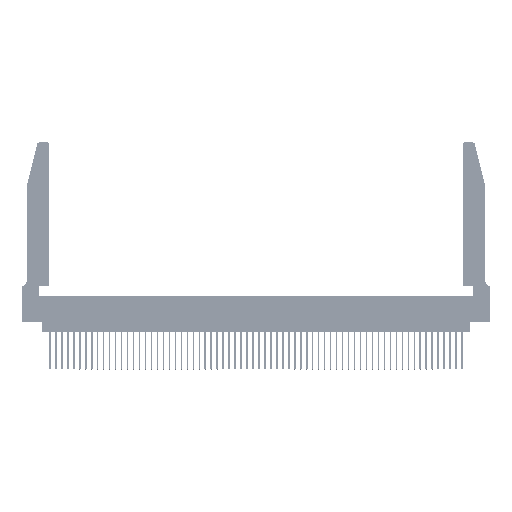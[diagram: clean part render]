
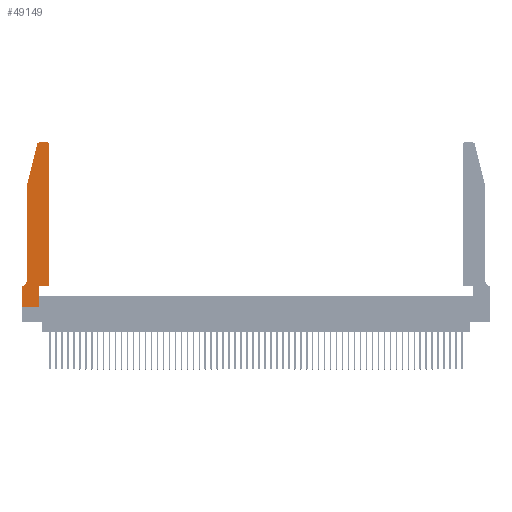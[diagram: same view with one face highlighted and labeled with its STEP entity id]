
A CAD part, top view. The second image highlights one B-rep face of the part: STEP entity #49149.
In plain terms, the highlighted planar face has unit normal (0, 0, 1).
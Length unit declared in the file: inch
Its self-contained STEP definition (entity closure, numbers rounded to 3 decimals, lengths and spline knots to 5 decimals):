
#308 = LINE ( 'NONE', #42443, #46411 ) ;
#454 = EDGE_CURVE ( 'NONE', #34632, #51511, #42920, .T. ) ;
#538 = LINE ( 'NONE', #3701, #51428 ) ;
#749 = EDGE_CURVE ( 'NONE', #15492, #6159, #21286, .T. ) ;
#1790 = CARTESIAN_POINT ( 'NONE',  ( 0.4205, 2.72, 0.37 ) ) ;
#1946 = DIRECTION ( 'NONE',  ( 1., 0., 0. ) ) ;
#1961 = VECTOR ( 'NONE', #26047, 39.37008 ) ;
#2184 = AXIS2_PLACEMENT_3D ( 'NONE', #32062, #45126, #1946 ) ;
#2428 = CARTESIAN_POINT ( 'NONE',  ( 0., 0.35, 0.37 ) ) ;
#2936 = FACE_OUTER_BOUND ( 'NONE', #8441, .T. ) ;
#3701 = CARTESIAN_POINT ( 'NONE',  ( 0., 0., 0.37 ) ) ;
#4046 = ORIENTED_EDGE ( 'NONE', *, *, #21004, .T. ) ;
#4963 = DIRECTION ( 'NONE',  ( -1., 0., 0. ) ) ;
#6159 = VERTEX_POINT ( 'NONE', #52684 ) ;
#6370 = VERTEX_POINT ( 'NONE', #18988 ) ;
#6462 = CIRCLE ( 'NONE', #9259, 0.03 ) ;
#6518 = ORIENTED_EDGE ( 'NONE', *, *, #55956, .T. ) ;
#6593 = CIRCLE ( 'NONE', #7332, 0.07 ) ;
#7332 = AXIS2_PLACEMENT_3D ( 'NONE', #45254, #49633, #28563 ) ;
#8377 = CARTESIAN_POINT ( 'NONE',  ( 0.0755, 2., 0.37 ) ) ;
#8441 = EDGE_LOOP ( 'NONE', ( #33001, #18082, #33596, #13042, #40337, #54365, #6518, #4046, #44190, #26264, #25350, #10329 ) ) ;
#9259 = AXIS2_PLACEMENT_3D ( 'NONE', #1790, #28641, #28462 ) ;
#10329 = ORIENTED_EDGE ( 'NONE', *, *, #38679, .T. ) ;
#11147 = VERTEX_POINT ( 'NONE', #2428 ) ;
#12492 = CARTESIAN_POINT ( 'NONE',  ( 0.0755, 2., 0.37 ) ) ;
#13042 = ORIENTED_EDGE ( 'NONE', *, *, #749, .T. ) ;
#13101 = EDGE_CURVE ( 'NONE', #50564, #11147, #18239, .T. ) ;
#14091 = DIRECTION ( 'NONE',  ( 0., 0., 1. ) ) ;
#14853 = CARTESIAN_POINT ( 'NONE',  ( 0.0755, 2., 0.37 ) ) ;
#15492 = VERTEX_POINT ( 'NONE', #12492 ) ;
#17785 = CARTESIAN_POINT ( 'NONE',  ( 0.4505, 0.35, 0.37 ) ) ;
#17996 = AXIS2_PLACEMENT_3D ( 'NONE', #18849, #14091, #49141 ) ;
#18082 = ORIENTED_EDGE ( 'NONE', *, *, #454, .T. ) ;
#18239 = LINE ( 'NONE', #39400, #41235 ) ;
#18849 = CARTESIAN_POINT ( 'NONE',  ( 0.284, 2.72, 0.37 ) ) ;
#18988 = CARTESIAN_POINT ( 'NONE',  ( 0.2865, 0.35, 0.37 ) ) ;
#20338 = DIRECTION ( 'NONE',  ( 0., 1., 0. ) ) ;
#21004 = EDGE_CURVE ( 'NONE', #37998, #21715, #23641, .T. ) ;
#21286 = LINE ( 'NONE', #8377, #32148 ) ;
#21448 = CARTESIAN_POINT ( 'NONE',  ( 0.4505, 2.72, 0.37 ) ) ;
#21715 = VERTEX_POINT ( 'NONE', #52553 ) ;
#23641 = LINE ( 'NONE', #29854, #1961 ) ;
#23735 = DIRECTION ( 'NONE',  ( -0.239, -0.971, 0. ) ) ;
#24909 = LINE ( 'NONE', #42332, #50003 ) ;
#25350 = ORIENTED_EDGE ( 'NONE', *, *, #33210, .T. ) ;
#25373 = CARTESIAN_POINT ( 'NONE',  ( 0.4205, 2.75, 0.37 ) ) ;
#25662 = VERTEX_POINT ( 'NONE', #25373 ) ;
#26047 = DIRECTION ( 'NONE',  ( 1., 0., 0. ) ) ;
#26264 = ORIENTED_EDGE ( 'NONE', *, *, #28695, .T. ) ;
#26743 = LINE ( 'NONE', #14853, #49842 ) ;
#28462 = DIRECTION ( 'NONE',  ( 1., 0., 0. ) ) ;
#28563 = DIRECTION ( 'NONE',  ( -1., 0., 0. ) ) ;
#28641 = DIRECTION ( 'NONE',  ( 0., 0., 1. ) ) ;
#28695 = EDGE_CURVE ( 'NONE', #6370, #44546, #34144, .T. ) ;
#29854 = CARTESIAN_POINT ( 'NONE',  ( 0., 0., 0.37 ) ) ;
#29981 = DIRECTION ( 'NONE',  ( 0., -1., 0. ) ) ;
#30315 = DIRECTION ( 'NONE',  ( 0., -1., 0. ) ) ;
#31941 = LINE ( 'NONE', #37715, #55636 ) ;
#32062 = CARTESIAN_POINT ( 'NONE',  ( 0., 0.35, 0.37 ) ) ;
#32148 = VECTOR ( 'NONE', #30315, 39.37008 ) ;
#32847 = DIRECTION ( 'NONE',  ( 1., 0., 0. ) ) ;
#33001 = ORIENTED_EDGE ( 'NONE', *, *, #38830, .T. ) ;
#33210 = EDGE_CURVE ( 'NONE', #44546, #39086, #24909, .T. ) ;
#33596 = ORIENTED_EDGE ( 'NONE', *, *, #38611, .T. ) ;
#33680 = CARTESIAN_POINT ( 'NONE',  ( 0.284, 2.75, 0.37 ) ) ;
#33989 = DIRECTION ( 'NONE',  ( 0., 1., 0. ) ) ;
#34144 = LINE ( 'NONE', #54081, #54491 ) ;
#34632 = VERTEX_POINT ( 'NONE', #33680 ) ;
#35718 = CARTESIAN_POINT ( 'NONE',  ( 0., 0., 0.37 ) ) ;
#37715 = CARTESIAN_POINT ( 'NONE',  ( 0.2865, 0.35, 0.37 ) ) ;
#37998 = VERTEX_POINT ( 'NONE', #35718 ) ;
#38611 = EDGE_CURVE ( 'NONE', #51511, #15492, #26743, .T. ) ;
#38679 = EDGE_CURVE ( 'NONE', #39086, #25662, #6462, .T. ) ;
#38830 = EDGE_CURVE ( 'NONE', #25662, #34632, #308, .T. ) ;
#39086 = VERTEX_POINT ( 'NONE', #21448 ) ;
#39400 = CARTESIAN_POINT ( 'NONE',  ( 0.0755, 0.35, 0.37 ) ) ;
#40337 = ORIENTED_EDGE ( 'NONE', *, *, #44007, .T. ) ;
#40708 = EDGE_CURVE ( 'NONE', #21715, #6370, #31941, .T. ) ;
#41122 = PLANE ( 'NONE',  #2184 ) ;
#41235 = VECTOR ( 'NONE', #4963, 39.37008 ) ;
#42332 = CARTESIAN_POINT ( 'NONE',  ( 0.4505, 0.35, 0.37 ) ) ;
#42443 = CARTESIAN_POINT ( 'NONE',  ( 0.2605, 2.75, 0.37 ) ) ;
#42920 = CIRCLE ( 'NONE', #17996, 0.03 ) ;
#44007 = EDGE_CURVE ( 'NONE', #6159, #50564, #6593, .T. ) ;
#44190 = ORIENTED_EDGE ( 'NONE', *, *, #40708, .T. ) ;
#44546 = VERTEX_POINT ( 'NONE', #17785 ) ;
#45126 = DIRECTION ( 'NONE',  ( 0., 0., 1. ) ) ;
#45254 = CARTESIAN_POINT ( 'NONE',  ( 0.0055, 0.42, 0.37 ) ) ;
#45481 = CARTESIAN_POINT ( 'NONE',  ( 0.0055, 0.35, 0.37 ) ) ;
#46411 = VECTOR ( 'NONE', #55536, 39.37008 ) ;
#47680 = CARTESIAN_POINT ( 'NONE',  ( 0.25487, 2.72718, 0.37 ) ) ;
#49141 = DIRECTION ( 'NONE',  ( 1., 0., 0. ) ) ;
#49149 = ADVANCED_FACE ( 'NONE', ( #2936 ), #41122, .T. ) ;
#49633 = DIRECTION ( 'NONE',  ( 0., 0., -1. ) ) ;
#49842 = VECTOR ( 'NONE', #23735, 39.37008 ) ;
#50003 = VECTOR ( 'NONE', #33989, 39.37008 ) ;
#50564 = VERTEX_POINT ( 'NONE', #45481 ) ;
#51428 = VECTOR ( 'NONE', #29981, 39.37008 ) ;
#51511 = VERTEX_POINT ( 'NONE', #47680 ) ;
#52553 = CARTESIAN_POINT ( 'NONE',  ( 0.2865, 0., 0.37 ) ) ;
#52684 = CARTESIAN_POINT ( 'NONE',  ( 0.0755, 0.42, 0.37 ) ) ;
#54081 = CARTESIAN_POINT ( 'NONE',  ( 0.4505, 0.35, 0.37 ) ) ;
#54365 = ORIENTED_EDGE ( 'NONE', *, *, #13101, .T. ) ;
#54491 = VECTOR ( 'NONE', #32847, 39.37008 ) ;
#55536 = DIRECTION ( 'NONE',  ( -1., 0., 0. ) ) ;
#55636 = VECTOR ( 'NONE', #20338, 39.37008 ) ;
#55956 = EDGE_CURVE ( 'NONE', #11147, #37998, #538, .T. ) ;
